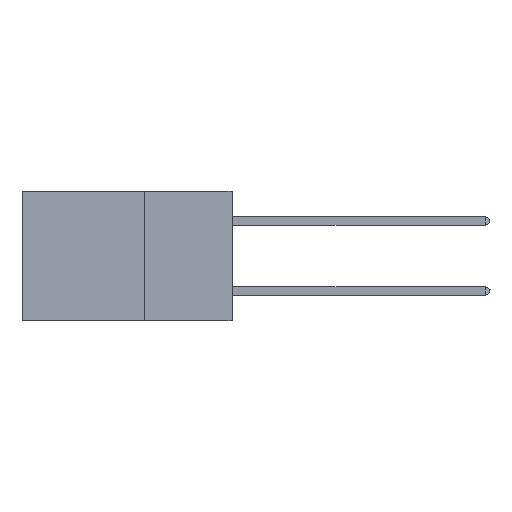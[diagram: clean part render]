
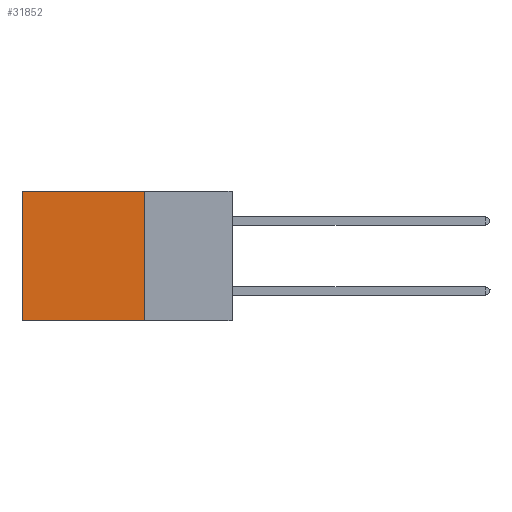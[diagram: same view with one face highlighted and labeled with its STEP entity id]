
A CAD part, left-side view. The second image highlights one B-rep face of the part: STEP entity #31852.
In plain terms, the highlighted planar face has unit normal (-1, 0, 0).
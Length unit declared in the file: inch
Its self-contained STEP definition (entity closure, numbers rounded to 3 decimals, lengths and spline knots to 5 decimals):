
#39 = CARTESIAN_POINT ( 'NONE',  ( 0.2875, 0.6, 0. ) ) ;
#1409 = LINE ( 'NONE', #8637, #6944 ) ;
#3917 = VERTEX_POINT ( 'NONE', #37940 ) ;
#4006 = DIRECTION ( 'NONE',  ( 1., 0., 0. ) ) ;
#5575 = ORIENTED_EDGE ( 'NONE', *, *, #29965, .T. ) ;
#6197 = VECTOR ( 'NONE', #23551, 39.37008 ) ;
#6944 = VECTOR ( 'NONE', #32372, 39.37008 ) ;
#8637 = CARTESIAN_POINT ( 'NONE',  ( 0.2875, 0.25, -0.37 ) ) ;
#8662 = DIRECTION ( 'NONE',  ( 0., 0., -1. ) ) ;
#10354 = CARTESIAN_POINT ( 'NONE',  ( 0.2875, 0.25, 0. ) ) ;
#11171 = ORIENTED_EDGE ( 'NONE', *, *, #20407, .F. ) ;
#11296 = ORIENTED_EDGE ( 'NONE', *, *, #37436, .T. ) ;
#12780 = VERTEX_POINT ( 'NONE', #38959 ) ;
#13135 = CARTESIAN_POINT ( 'NONE',  ( 0.2875, 0.25, -0.37 ) ) ;
#14278 = CARTESIAN_POINT ( 'NONE',  ( 0.2875, 0.6, 0. ) ) ;
#15384 = VERTEX_POINT ( 'NONE', #39 ) ;
#17541 = VERTEX_POINT ( 'NONE', #13135 ) ;
#19321 = EDGE_LOOP ( 'NONE', ( #5575, #11171, #37645, #11296 ) ) ;
#20282 = CARTESIAN_POINT ( 'NONE',  ( 0.2875, 0.25, 0. ) ) ;
#20407 = EDGE_CURVE ( 'NONE', #17541, #3917, #1409, .T. ) ;
#23355 = LINE ( 'NONE', #20282, #6197 ) ;
#23551 = DIRECTION ( 'NONE',  ( 0., 1., 0. ) ) ;
#23650 = LINE ( 'NONE', #14278, #39925 ) ;
#24377 = LINE ( 'NONE', #27872, #41121 ) ;
#26005 = FACE_OUTER_BOUND ( 'NONE', #19321, .T. ) ;
#27872 = CARTESIAN_POINT ( 'NONE',  ( 0.2875, 0.25, 0. ) ) ;
#29965 = EDGE_CURVE ( 'NONE', #15384, #3917, #23650, .T. ) ;
#31852 = ADVANCED_FACE ( 'NONE', ( #26005 ), #35980, .F. ) ;
#32372 = DIRECTION ( 'NONE',  ( 0., 1., 0. ) ) ;
#33393 = EDGE_CURVE ( 'NONE', #12780, #17541, #24377, .T. ) ;
#33461 = AXIS2_PLACEMENT_3D ( 'NONE', #10354, #4006, #36122 ) ;
#35980 = PLANE ( 'NONE',  #33461 ) ;
#36122 = DIRECTION ( 'NONE',  ( 0., 0., -1. ) ) ;
#37436 = EDGE_CURVE ( 'NONE', #12780, #15384, #23355, .T. ) ;
#37645 = ORIENTED_EDGE ( 'NONE', *, *, #33393, .F. ) ;
#37940 = CARTESIAN_POINT ( 'NONE',  ( 0.2875, 0.6, -0.37 ) ) ;
#38959 = CARTESIAN_POINT ( 'NONE',  ( 0.2875, 0.25, 0. ) ) ;
#39925 = VECTOR ( 'NONE', #40092, 39.37008 ) ;
#40092 = DIRECTION ( 'NONE',  ( 0., 0., -1. ) ) ;
#41121 = VECTOR ( 'NONE', #8662, 39.37008 ) ;
